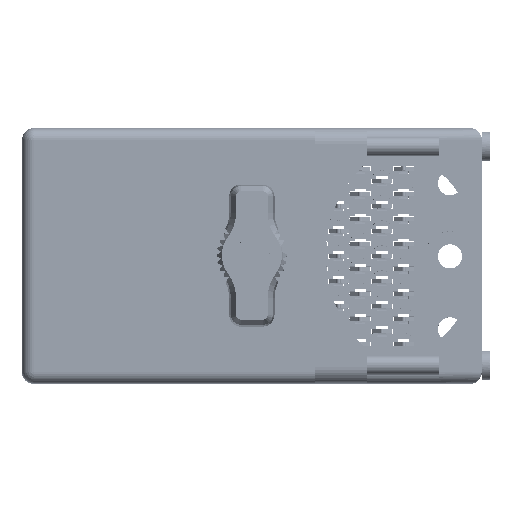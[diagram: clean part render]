
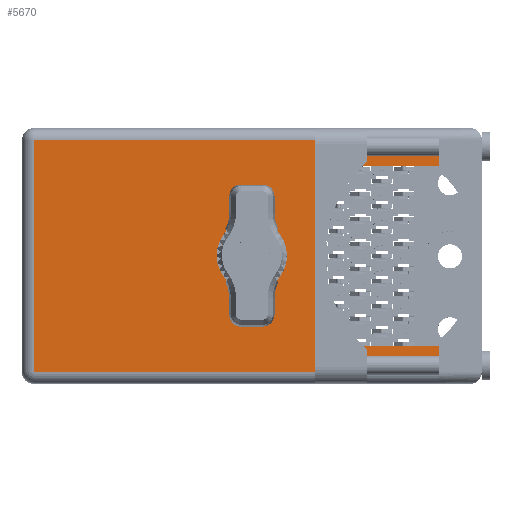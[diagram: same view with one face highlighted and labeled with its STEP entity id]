
A CAD part, top view. The second image highlights one B-rep face of the part: STEP entity #5670.
In plain terms, the highlighted face is planar.
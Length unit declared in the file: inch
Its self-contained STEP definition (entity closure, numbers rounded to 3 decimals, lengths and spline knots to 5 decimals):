
#854 = DIRECTION ( 'NONE',  ( -1., 0., 0. ) ) ;
#1146 = EDGE_CURVE ( 'NONE', #24750, #6638, #27092, .T. ) ;
#2612 = CARTESIAN_POINT ( 'NONE',  ( 1.1215, 1.93, 0.54 ) ) ;
#3789 = CARTESIAN_POINT ( 'NONE',  ( 0.4075, 1.93, -0.54 ) ) ;
#4433 = ORIENTED_EDGE ( 'NONE', *, *, #46865, .F. ) ;
#5670 = ADVANCED_FACE ( 'NONE', ( #54196, #73386 ), #101448, .T. ) ;
#6638 = VERTEX_POINT ( 'NONE', #64512 ) ;
#8938 = AXIS2_PLACEMENT_3D ( 'NONE', #60798, #28331, #69022 ) ;
#11175 = VECTOR ( 'NONE', #71771, 39.37008 ) ;
#12270 = LINE ( 'NONE', #89607, #96582 ) ;
#13208 = CARTESIAN_POINT ( 'NONE',  ( 1.1215, 1.93, -0.695 ) ) ;
#19640 = VERTEX_POINT ( 'NONE', #99890 ) ;
#22098 = DIRECTION ( 'NONE',  ( 0., 0., 1. ) ) ;
#23453 = EDGE_LOOP ( 'NONE', ( #80481, #4433 ) ) ;
#24358 = CARTESIAN_POINT ( 'NONE',  ( 1.1215, 1.93, -0.765 ) ) ;
#24750 = VERTEX_POINT ( 'NONE', #2612 ) ;
#25460 = VERTEX_POINT ( 'NONE', #77808 ) ;
#27092 = LINE ( 'NONE', #64678, #98558 ) ;
#28192 = ORIENTED_EDGE ( 'NONE', *, *, #50713, .T. ) ;
#28256 = CARTESIAN_POINT ( 'NONE',  ( 0.4075, 1.93, -0.54 ) ) ;
#28331 = DIRECTION ( 'NONE',  ( 0., 1., 0. ) ) ;
#30183 = ORIENTED_EDGE ( 'NONE', *, *, #63913, .T. ) ;
#34730 = ORIENTED_EDGE ( 'NONE', *, *, #1146, .T. ) ;
#36394 = AXIS2_PLACEMENT_3D ( 'NONE', #53037, #69489, #37010 ) ;
#37010 = DIRECTION ( 'NONE',  ( 0., 0., 1. ) ) ;
#38677 = EDGE_LOOP ( 'NONE', ( #30183, #74220, #49766, #34730, #28192, #42181, #73659, #48455 ) ) ;
#40390 = LINE ( 'NONE', #90415, #94066 ) ;
#40697 = DIRECTION ( 'NONE',  ( 1., 0., 0. ) ) ;
#42181 = ORIENTED_EDGE ( 'NONE', *, *, #56059, .T. ) ;
#42228 = LINE ( 'NONE', #24358, #61356 ) ;
#44470 = VECTOR ( 'NONE', #50860, 39.37008 ) ;
#46750 = DIRECTION ( 'NONE',  ( 0., 1., 0. ) ) ;
#46865 = EDGE_CURVE ( 'NONE', #72922, #25460, #60253, .T. ) ;
#48455 = ORIENTED_EDGE ( 'NONE', *, *, #94642, .T. ) ;
#48724 = VERTEX_POINT ( 'NONE', #13208 ) ;
#49766 = ORIENTED_EDGE ( 'NONE', *, *, #67106, .F. ) ;
#50713 = EDGE_CURVE ( 'NONE', #6638, #51866, #92801, .T. ) ;
#50860 = DIRECTION ( 'NONE',  ( 0., 0., 1. ) ) ;
#51658 = VERTEX_POINT ( 'NONE', #90589 ) ;
#51866 = VERTEX_POINT ( 'NONE', #3789 ) ;
#53037 = CARTESIAN_POINT ( 'NONE',  ( 0., 1.93, 0. ) ) ;
#53667 = EDGE_CURVE ( 'NONE', #25460, #72922, #70589, .T. ) ;
#54196 = FACE_OUTER_BOUND ( 'NONE', #38677, .T. ) ;
#56059 = EDGE_CURVE ( 'NONE', #51866, #51658, #102167, .T. ) ;
#56223 = EDGE_CURVE ( 'NONE', #48724, #51658, #42228, .T. ) ;
#56255 = CARTESIAN_POINT ( 'NONE',  ( -1.3075, 1.93, -0.695 ) ) ;
#57527 = DIRECTION ( 'NONE',  ( 0., 0., 1. ) ) ;
#60253 = CIRCLE ( 'NONE', #91290, 0.17 ) ;
#60798 = CARTESIAN_POINT ( 'NONE',  ( -1.3775, 1.93, -0.765 ) ) ;
#61356 = VECTOR ( 'NONE', #57527, 39.37008 ) ;
#63913 = EDGE_CURVE ( 'NONE', #75442, #66995, #97369, .T. ) ;
#64512 = CARTESIAN_POINT ( 'NONE',  ( 0.4075, 1.93, 0.54 ) ) ;
#64678 = CARTESIAN_POINT ( 'NONE',  ( 1.1215, 1.93, 0.54 ) ) ;
#64793 = CARTESIAN_POINT ( 'NONE',  ( 0., 1.93, -0.17 ) ) ;
#65748 = DIRECTION ( 'NONE',  ( -1., 0., 0. ) ) ;
#66188 = LINE ( 'NONE', #74433, #44470 ) ;
#66995 = VERTEX_POINT ( 'NONE', #90530 ) ;
#67106 = EDGE_CURVE ( 'NONE', #24750, #19640, #66188, .T. ) ;
#68182 = EDGE_CURVE ( 'NONE', #66995, #19640, #12270, .T. ) ;
#69022 = DIRECTION ( 'NONE',  ( -1., 0., 0. ) ) ;
#69489 = DIRECTION ( 'NONE',  ( 0., 1., 0. ) ) ;
#70589 = CIRCLE ( 'NONE', #36394, 0.17 ) ;
#71771 = DIRECTION ( 'NONE',  ( 0., 0., -1. ) ) ;
#72922 = VERTEX_POINT ( 'NONE', #64793 ) ;
#73386 = FACE_BOUND ( 'NONE', #23453, .T. ) ;
#73659 = ORIENTED_EDGE ( 'NONE', *, *, #56223, .F. ) ;
#74220 = ORIENTED_EDGE ( 'NONE', *, *, #68182, .T. ) ;
#74433 = CARTESIAN_POINT ( 'NONE',  ( 1.1215, 1.93, -0.765 ) ) ;
#75442 = VERTEX_POINT ( 'NONE', #56255 ) ;
#77808 = CARTESIAN_POINT ( 'NONE',  ( 0., 1.93, 0.17 ) ) ;
#79578 = CARTESIAN_POINT ( 'NONE',  ( -1.3075, 1.93, -0.765 ) ) ;
#80481 = ORIENTED_EDGE ( 'NONE', *, *, #53667, .F. ) ;
#82011 = VECTOR ( 'NONE', #22098, 39.37008 ) ;
#88281 = DIRECTION ( 'NONE',  ( 1., 0., 0. ) ) ;
#89345 = CARTESIAN_POINT ( 'NONE',  ( 1.1215, 1.93, -0.54 ) ) ;
#89607 = CARTESIAN_POINT ( 'NONE',  ( 1.1215, 1.93, 0.695 ) ) ;
#90415 = CARTESIAN_POINT ( 'NONE',  ( -1.3775, 1.93, -0.695 ) ) ;
#90530 = CARTESIAN_POINT ( 'NONE',  ( -1.3075, 1.93, 0.695 ) ) ;
#90589 = CARTESIAN_POINT ( 'NONE',  ( 1.1215, 1.93, -0.54 ) ) ;
#91290 = AXIS2_PLACEMENT_3D ( 'NONE', #95994, #46750, #95291 ) ;
#92801 = LINE ( 'NONE', #28256, #11175 ) ;
#94066 = VECTOR ( 'NONE', #854, 39.37008 ) ;
#94642 = EDGE_CURVE ( 'NONE', #48724, #75442, #40390, .T. ) ;
#95291 = DIRECTION ( 'NONE',  ( 0., 0., 1. ) ) ;
#95994 = CARTESIAN_POINT ( 'NONE',  ( 0., 1.93, 0. ) ) ;
#96582 = VECTOR ( 'NONE', #40697, 39.37008 ) ;
#97103 = VECTOR ( 'NONE', #88281, 39.37008 ) ;
#97369 = LINE ( 'NONE', #79578, #82011 ) ;
#98558 = VECTOR ( 'NONE', #65748, 39.37008 ) ;
#99890 = CARTESIAN_POINT ( 'NONE',  ( 1.1215, 1.93, 0.695 ) ) ;
#101448 = PLANE ( 'NONE',  #8938 ) ;
#102167 = LINE ( 'NONE', #89345, #97103 ) ;
